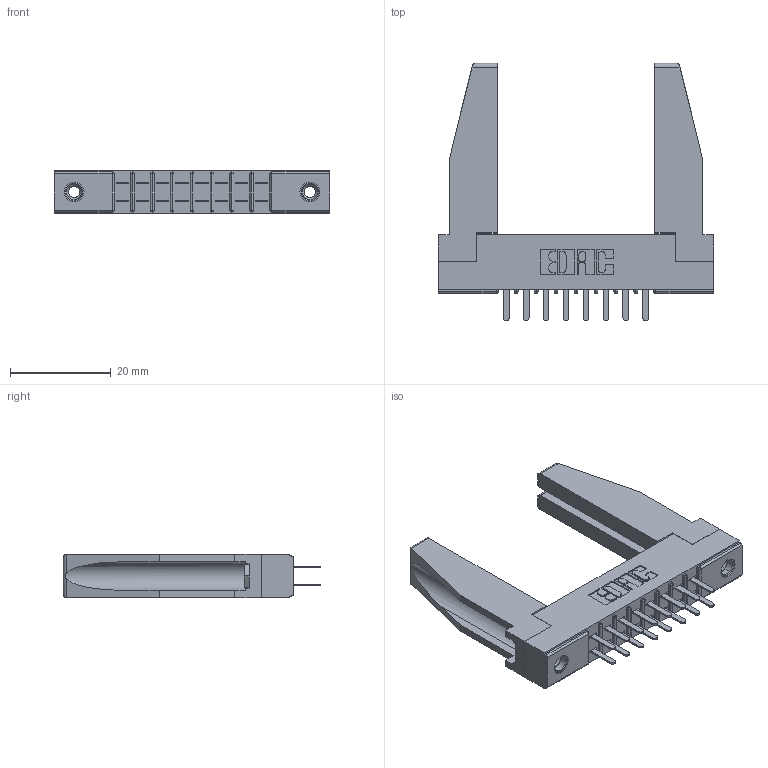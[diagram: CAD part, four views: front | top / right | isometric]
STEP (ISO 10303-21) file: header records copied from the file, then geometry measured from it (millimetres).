
FILE_DESCRIPTION (( 'STEP AP203' ), '1' );
FILE_NAME ('305-016-520-278.STEP', '2019-09-09T12:10:26', ( '' ), ( '' ), 'SwSTEP 2.0', 'SolidWorks 2016', '' );
FILE_SCHEMA (( 'CONFIG_CONTROL_DESIGN' ));
Length unit declared in the file: inch
Products named in the file (5): 307-220-078; 305-016-520-278; 305 Part_.156 Dia; 305-290-001_520; 345-250-001_345-250-001-102
Assembly tree (21 placements, depth 2):
  305-016-520-278
    305 Part_.156 Dia
    305-290-001_520  x16
    345-250-001_345-250-001-102  x2
    307-220-078  x2
Bounding box: 54.71 x 51.13 x 8.71 mm (x, y, z)
Volume: 7440.7 mm3; surface area: 9534 mm2
Topology: 21 solids, 21 shells, 982 faces, 2750 edges, 1780 vertices
Faces by surface type: plane 584, cylinder 350, sphere 32, cone 12, torus 4
Entity records: 15120 total; most frequent: CARTESIAN_POINT 2508, ORIENTED_EDGE 2442, DIRECTION 2411, EDGE_CURVE 1221, VECTOR 949, LINE 949, VERTEX_POINT 786, AXIS2_PLACEMENT_3D 731
